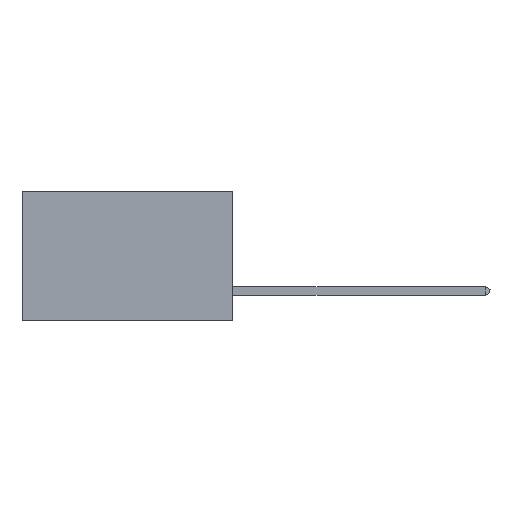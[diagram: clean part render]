
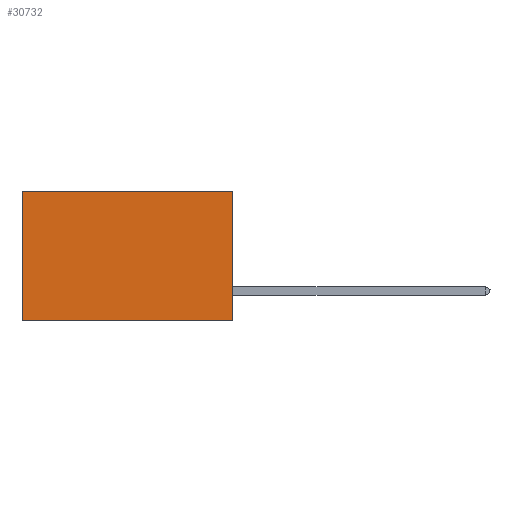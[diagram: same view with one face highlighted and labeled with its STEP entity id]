
A CAD part, left-side view. The second image highlights one B-rep face of the part: STEP entity #30732.
In plain terms, the highlighted planar face has unit normal (-1, 0, 0).
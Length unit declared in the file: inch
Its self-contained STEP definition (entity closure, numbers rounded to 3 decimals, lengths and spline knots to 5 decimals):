
#1870 = PLANE ( 'NONE',  #18002 ) ;
#3091 = LINE ( 'NONE', #41550, #15407 ) ;
#5659 = CARTESIAN_POINT ( 'NONE',  ( 0.2875, 0., 0. ) ) ;
#8455 = EDGE_CURVE ( 'NONE', #25722, #39743, #32721, .T. ) ;
#11882 = EDGE_CURVE ( 'NONE', #13702, #44654, #3091, .T. ) ;
#13177 = DIRECTION ( 'NONE',  ( 0., 0., -1. ) ) ;
#13288 = CARTESIAN_POINT ( 'NONE',  ( 0.2875, 0.6, 0. ) ) ;
#13702 = VERTEX_POINT ( 'NONE', #37522 ) ;
#15190 = DIRECTION ( 'NONE',  ( 0., 0., -1. ) ) ;
#15407 = VECTOR ( 'NONE', #26915, 39.37008 ) ;
#16483 = VECTOR ( 'NONE', #15190, 39.37008 ) ;
#16773 = ORIENTED_EDGE ( 'NONE', *, *, #39947, .F. ) ;
#18002 = AXIS2_PLACEMENT_3D ( 'NONE', #5659, #35623, #13177 ) ;
#21304 = CARTESIAN_POINT ( 'NONE',  ( 0.2875, 0., 0. ) ) ;
#21378 = ORIENTED_EDGE ( 'NONE', *, *, #11882, .F. ) ;
#22040 = FACE_OUTER_BOUND ( 'NONE', #24980, .T. ) ;
#22141 = EDGE_CURVE ( 'NONE', #39743, #44654, #32311, .T. ) ;
#24980 = EDGE_LOOP ( 'NONE', ( #37774, #21378, #16773, #36582 ) ) ;
#25722 = VERTEX_POINT ( 'NONE', #27587 ) ;
#26915 = DIRECTION ( 'NONE',  ( 0., 1., 0. ) ) ;
#27587 = CARTESIAN_POINT ( 'NONE',  ( 0.2875, 0., 0. ) ) ;
#29479 = DIRECTION ( 'NONE',  ( 0., 0., -1. ) ) ;
#29483 = VECTOR ( 'NONE', #29479, 39.37008 ) ;
#30732 = ADVANCED_FACE ( 'NONE', ( #22040 ), #1870, .F. ) ;
#32311 = LINE ( 'NONE', #45090, #16483 ) ;
#32721 = LINE ( 'NONE', #46538, #35081 ) ;
#34367 = CARTESIAN_POINT ( 'NONE',  ( 0.2875, 0.6, -0.37 ) ) ;
#35081 = VECTOR ( 'NONE', #35588, 39.37008 ) ;
#35588 = DIRECTION ( 'NONE',  ( 0., 1., 0. ) ) ;
#35623 = DIRECTION ( 'NONE',  ( 1., 0., 0. ) ) ;
#36582 = ORIENTED_EDGE ( 'NONE', *, *, #8455, .T. ) ;
#37522 = CARTESIAN_POINT ( 'NONE',  ( 0.2875, 0., -0.37 ) ) ;
#37774 = ORIENTED_EDGE ( 'NONE', *, *, #22141, .T. ) ;
#39500 = LINE ( 'NONE', #21304, #29483 ) ;
#39743 = VERTEX_POINT ( 'NONE', #13288 ) ;
#39947 = EDGE_CURVE ( 'NONE', #25722, #13702, #39500, .T. ) ;
#41550 = CARTESIAN_POINT ( 'NONE',  ( 0.2875, 0., -0.37 ) ) ;
#44654 = VERTEX_POINT ( 'NONE', #34367 ) ;
#45090 = CARTESIAN_POINT ( 'NONE',  ( 0.2875, 0.6, 0. ) ) ;
#46538 = CARTESIAN_POINT ( 'NONE',  ( 0.2875, 0., 0. ) ) ;
